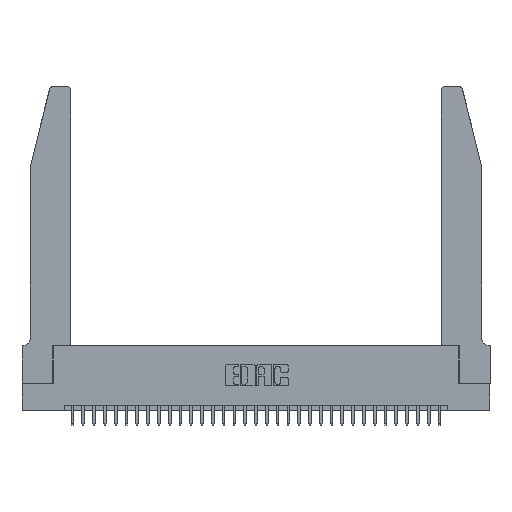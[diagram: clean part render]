
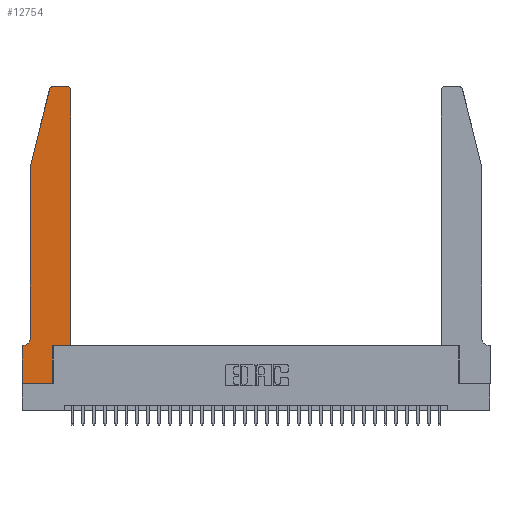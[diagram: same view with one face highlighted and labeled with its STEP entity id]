
A CAD part, top view. The second image highlights one B-rep face of the part: STEP entity #12754.
In plain terms, the highlighted planar face has unit normal (0, 0, 1).
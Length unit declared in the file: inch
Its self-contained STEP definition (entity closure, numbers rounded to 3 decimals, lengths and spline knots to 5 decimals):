
#39 = ORIENTED_EDGE ( 'NONE', *, *, #15829, .T. ) ;
#354 = DIRECTION ( 'NONE',  ( 0., -1., 0. ) ) ;
#393 = DIRECTION ( 'NONE',  ( 0., 1., 0. ) ) ;
#442 = EDGE_LOOP ( 'NONE', ( #21399, #19911, #24892, #20730, #8486, #39, #29328, #23375, #21958, #21159, #9276, #19694 ) ) ;
#1120 = LINE ( 'NONE', #16913, #28333 ) ;
#1558 = EDGE_CURVE ( 'NONE', #6648, #25429, #18327, .T. ) ;
#1687 = VECTOR ( 'NONE', #32110, 39.37008 ) ;
#2188 = EDGE_CURVE ( 'NONE', #12480, #20342, #11929, .T. ) ;
#4004 = CARTESIAN_POINT ( 'NONE',  ( 0.0755, 2., 0.37 ) ) ;
#4684 = CARTESIAN_POINT ( 'NONE',  ( 0., 0.35, 0.37 ) ) ;
#5292 = LINE ( 'NONE', #15314, #18026 ) ;
#5734 = DIRECTION ( 'NONE',  ( 1., 0., 0. ) ) ;
#5898 = CARTESIAN_POINT ( 'NONE',  ( 0.284, 2.72, 0.37 ) ) ;
#6267 = VECTOR ( 'NONE', #8946, 39.37008 ) ;
#6648 = VERTEX_POINT ( 'NONE', #29314 ) ;
#7030 = CARTESIAN_POINT ( 'NONE',  ( 0.0755, 0.35, 0.37 ) ) ;
#7295 = PLANE ( 'NONE',  #22886 ) ;
#8482 = DIRECTION ( 'NONE',  ( 1., 0., 0. ) ) ;
#8486 = ORIENTED_EDGE ( 'NONE', *, *, #15973, .T. ) ;
#8946 = DIRECTION ( 'NONE',  ( 0., 1., 0. ) ) ;
#9276 = ORIENTED_EDGE ( 'NONE', *, *, #23794, .T. ) ;
#9550 = CARTESIAN_POINT ( 'NONE',  ( 0.25487, 2.72718, 0.37 ) ) ;
#9588 = DIRECTION ( 'NONE',  ( -1., 0., 0. ) ) ;
#9848 = DIRECTION ( 'NONE',  ( 1., 0., 0. ) ) ;
#10046 = VERTEX_POINT ( 'NONE', #22862 ) ;
#10142 = DIRECTION ( 'NONE',  ( 0., 0., -1. ) ) ;
#10563 = VECTOR ( 'NONE', #9588, 39.37008 ) ;
#11100 = DIRECTION ( 'NONE',  ( 0., 0., 1. ) ) ;
#11719 = CIRCLE ( 'NONE', #21671, 0.03 ) ;
#11929 = LINE ( 'NONE', #31069, #24636 ) ;
#11932 = EDGE_CURVE ( 'NONE', #20997, #6648, #27499, .T. ) ;
#12350 = DIRECTION ( 'NONE',  ( 0., -1., 0. ) ) ;
#12480 = VERTEX_POINT ( 'NONE', #26292 ) ;
#12754 = ADVANCED_FACE ( 'NONE', ( #31491 ), #7295, .T. ) ;
#13295 = CIRCLE ( 'NONE', #27410, 0.07 ) ;
#13823 = LINE ( 'NONE', #26708, #6267 ) ;
#14023 = LINE ( 'NONE', #30176, #27549 ) ;
#14843 = DIRECTION ( 'NONE',  ( 0., 0., 1. ) ) ;
#15039 = VERTEX_POINT ( 'NONE', #23685 ) ;
#15314 = CARTESIAN_POINT ( 'NONE',  ( 0.2605, 2.75, 0.37 ) ) ;
#15424 = CARTESIAN_POINT ( 'NONE',  ( 0.2865, 0.35, 0.37 ) ) ;
#15527 = EDGE_CURVE ( 'NONE', #15039, #25201, #21664, .T. ) ;
#15829 = EDGE_CURVE ( 'NONE', #31798, #10046, #30875, .T. ) ;
#15973 = EDGE_CURVE ( 'NONE', #20342, #31798, #13295, .T. ) ;
#16532 = VERTEX_POINT ( 'NONE', #24628 ) ;
#16738 = EDGE_CURVE ( 'NONE', #16532, #15039, #5292, .T. ) ;
#16908 = LINE ( 'NONE', #4004, #1687 ) ;
#16913 = CARTESIAN_POINT ( 'NONE',  ( 0.4505, 0.35, 0.37 ) ) ;
#17539 = VECTOR ( 'NONE', #393, 39.37008 ) ;
#17846 = DIRECTION ( 'NONE',  ( -1., 0., 0. ) ) ;
#18026 = VECTOR ( 'NONE', #17846, 39.37008 ) ;
#18327 = LINE ( 'NONE', #18370, #17539 ) ;
#18370 = CARTESIAN_POINT ( 'NONE',  ( 0.2865, 0.35, 0.37 ) ) ;
#19501 = AXIS2_PLACEMENT_3D ( 'NONE', #5898, #23681, #8482 ) ;
#19694 = ORIENTED_EDGE ( 'NONE', *, *, #26876, .T. ) ;
#19902 = DIRECTION ( 'NONE',  ( 1., 0., 0. ) ) ;
#19911 = ORIENTED_EDGE ( 'NONE', *, *, #15527, .T. ) ;
#20342 = VERTEX_POINT ( 'NONE', #27625 ) ;
#20717 = VECTOR ( 'NONE', #5734, 39.37008 ) ;
#20730 = ORIENTED_EDGE ( 'NONE', *, *, #2188, .T. ) ;
#20997 = VERTEX_POINT ( 'NONE', #22458 ) ;
#21007 = EDGE_CURVE ( 'NONE', #10046, #20997, #14023, .T. ) ;
#21042 = CARTESIAN_POINT ( 'NONE',  ( 0.4505, 2.72, 0.37 ) ) ;
#21159 = ORIENTED_EDGE ( 'NONE', *, *, #28547, .T. ) ;
#21399 = ORIENTED_EDGE ( 'NONE', *, *, #16738, .T. ) ;
#21664 = CIRCLE ( 'NONE', #19501, 0.03 ) ;
#21671 = AXIS2_PLACEMENT_3D ( 'NONE', #26322, #11100, #28913 ) ;
#21958 = ORIENTED_EDGE ( 'NONE', *, *, #1558, .T. ) ;
#22096 = CARTESIAN_POINT ( 'NONE',  ( 0.0055, 0.35, 0.37 ) ) ;
#22458 = CARTESIAN_POINT ( 'NONE',  ( 0., 0., 0.37 ) ) ;
#22807 = CARTESIAN_POINT ( 'NONE',  ( 0.4505, 0.35, 0.37 ) ) ;
#22862 = CARTESIAN_POINT ( 'NONE',  ( 0., 0.35, 0.37 ) ) ;
#22886 = AXIS2_PLACEMENT_3D ( 'NONE', #4684, #14843, #9848 ) ;
#23375 = ORIENTED_EDGE ( 'NONE', *, *, #11932, .T. ) ;
#23412 = CARTESIAN_POINT ( 'NONE',  ( 0., 0., 0.37 ) ) ;
#23681 = DIRECTION ( 'NONE',  ( 0., 0., 1. ) ) ;
#23685 = CARTESIAN_POINT ( 'NONE',  ( 0.284, 2.75, 0.37 ) ) ;
#23794 = EDGE_CURVE ( 'NONE', #28666, #25584, #13823, .T. ) ;
#24628 = CARTESIAN_POINT ( 'NONE',  ( 0.4205, 2.75, 0.37 ) ) ;
#24636 = VECTOR ( 'NONE', #354, 39.37008 ) ;
#24892 = ORIENTED_EDGE ( 'NONE', *, *, #25761, .T. ) ;
#25201 = VERTEX_POINT ( 'NONE', #9550 ) ;
#25344 = CARTESIAN_POINT ( 'NONE',  ( 0.0055, 0.42, 0.37 ) ) ;
#25429 = VERTEX_POINT ( 'NONE', #15424 ) ;
#25584 = VERTEX_POINT ( 'NONE', #21042 ) ;
#25761 = EDGE_CURVE ( 'NONE', #25201, #12480, #16908, .T. ) ;
#26292 = CARTESIAN_POINT ( 'NONE',  ( 0.0755, 2., 0.37 ) ) ;
#26322 = CARTESIAN_POINT ( 'NONE',  ( 0.4205, 2.72, 0.37 ) ) ;
#26708 = CARTESIAN_POINT ( 'NONE',  ( 0.4505, 0.35, 0.37 ) ) ;
#26876 = EDGE_CURVE ( 'NONE', #25584, #16532, #11719, .T. ) ;
#27410 = AXIS2_PLACEMENT_3D ( 'NONE', #25344, #10142, #27907 ) ;
#27499 = LINE ( 'NONE', #23412, #20717 ) ;
#27549 = VECTOR ( 'NONE', #12350, 39.37008 ) ;
#27625 = CARTESIAN_POINT ( 'NONE',  ( 0.0755, 0.42, 0.37 ) ) ;
#27907 = DIRECTION ( 'NONE',  ( -1., 0., 0. ) ) ;
#28333 = VECTOR ( 'NONE', #19902, 39.37008 ) ;
#28547 = EDGE_CURVE ( 'NONE', #25429, #28666, #1120, .T. ) ;
#28666 = VERTEX_POINT ( 'NONE', #22807 ) ;
#28913 = DIRECTION ( 'NONE',  ( 1., 0., 0. ) ) ;
#29314 = CARTESIAN_POINT ( 'NONE',  ( 0.2865, 0., 0.37 ) ) ;
#29328 = ORIENTED_EDGE ( 'NONE', *, *, #21007, .T. ) ;
#30176 = CARTESIAN_POINT ( 'NONE',  ( 0., 0., 0.37 ) ) ;
#30875 = LINE ( 'NONE', #7030, #10563 ) ;
#31069 = CARTESIAN_POINT ( 'NONE',  ( 0.0755, 2., 0.37 ) ) ;
#31491 = FACE_OUTER_BOUND ( 'NONE', #442, .T. ) ;
#31798 = VERTEX_POINT ( 'NONE', #22096 ) ;
#32110 = DIRECTION ( 'NONE',  ( -0.239, -0.971, 0. ) ) ;
